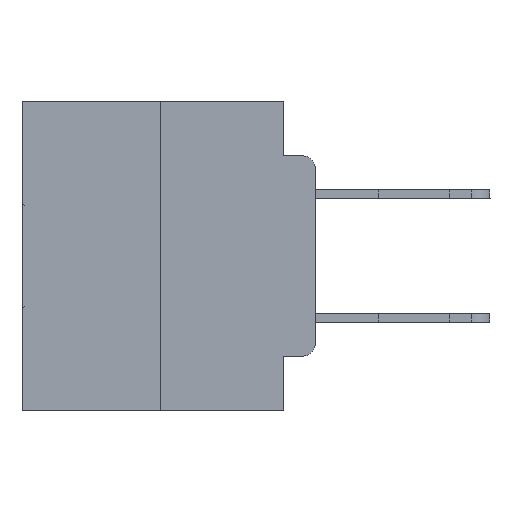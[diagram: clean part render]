
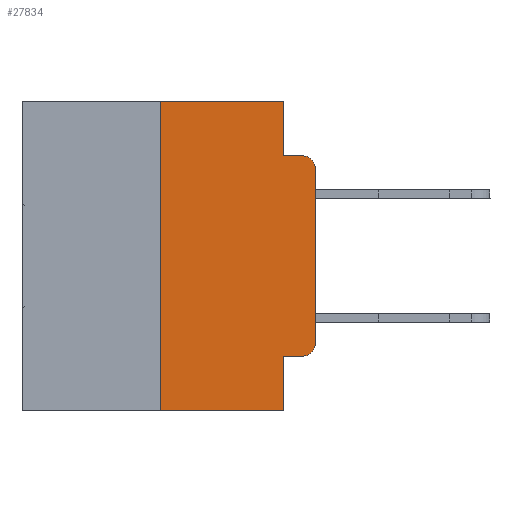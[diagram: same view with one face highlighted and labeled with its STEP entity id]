
A CAD part, left-side view. The second image highlights one B-rep face of the part: STEP entity #27834.
In plain terms, the highlighted planar face has unit normal (-1, 0, 0).
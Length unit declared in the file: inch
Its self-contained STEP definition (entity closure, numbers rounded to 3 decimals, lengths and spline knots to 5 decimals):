
#879 = ORIENTED_EDGE ( 'NONE', *, *, #26324, .F. ) ;
#1026 = FACE_OUTER_BOUND ( 'NONE', #24038, .T. ) ;
#1085 = DIRECTION ( 'NONE',  ( 0., -1., 0. ) ) ;
#1573 = CARTESIAN_POINT ( 'NONE',  ( 0., 0.051, -0.0885 ) ) ;
#1592 = CARTESIAN_POINT ( 'NONE',  ( 0., 0., 0. ) ) ;
#1932 = DIRECTION ( 'NONE',  ( 0., 0., -1. ) ) ;
#1944 = CARTESIAN_POINT ( 'NONE',  ( 0., 0.051, -0.5 ) ) ;
#1952 = CARTESIAN_POINT ( 'NONE',  ( 0., 0.25, -0.5 ) ) ;
#2003 = VERTEX_POINT ( 'NONE', #3719 ) ;
#2290 = VERTEX_POINT ( 'NONE', #1952 ) ;
#2358 = CARTESIAN_POINT ( 'NONE',  ( 0., 0.473, 0. ) ) ;
#2418 = LINE ( 'NONE', #1573, #20305 ) ;
#3221 = CARTESIAN_POINT ( 'NONE',  ( 0., 0.02, -0.4115 ) ) ;
#3252 = AXIS2_PLACEMENT_3D ( 'NONE', #21155, #7186, #23460 ) ;
#3294 = ORIENTED_EDGE ( 'NONE', *, *, #29349, .F. ) ;
#3719 = CARTESIAN_POINT ( 'NONE',  ( 0., 0.25, 0. ) ) ;
#3721 = ORIENTED_EDGE ( 'NONE', *, *, #3937, .F. ) ;
#3920 = DIRECTION ( 'NONE',  ( 0., 0., 1. ) ) ;
#3937 = EDGE_CURVE ( 'NONE', #16353, #20199, #2418, .T. ) ;
#4696 = DIRECTION ( 'NONE',  ( 0., 0., -1. ) ) ;
#5436 = ORIENTED_EDGE ( 'NONE', *, *, #29556, .F. ) ;
#5504 = CARTESIAN_POINT ( 'NONE',  ( 0., 0.02, -0.0885 ) ) ;
#5523 = EDGE_CURVE ( 'NONE', #25826, #20199, #20836, .T. ) ;
#5842 = VECTOR ( 'NONE', #9040, 39.37008 ) ;
#6154 = ORIENTED_EDGE ( 'NONE', *, *, #18633, .T. ) ;
#7186 = DIRECTION ( 'NONE',  ( -1., 0., 0. ) ) ;
#8644 = EDGE_CURVE ( 'NONE', #14102, #25826, #17054, .T. ) ;
#8721 = AXIS2_PLACEMENT_3D ( 'NONE', #29658, #15939, #1932 ) ;
#9040 = DIRECTION ( 'NONE',  ( 0., -1., 0. ) ) ;
#9070 = ORIENTED_EDGE ( 'NONE', *, *, #24800, .F. ) ;
#9284 = DIRECTION ( 'NONE',  ( 0., 0., -1. ) ) ;
#9444 = ORIENTED_EDGE ( 'NONE', *, *, #23275, .T. ) ;
#10222 = CARTESIAN_POINT ( 'NONE',  ( 0., 0.051, -0.4115 ) ) ;
#10243 = ORIENTED_EDGE ( 'NONE', *, *, #5523, .T. ) ;
#10339 = CARTESIAN_POINT ( 'NONE',  ( 0., 0., -0.3915 ) ) ;
#10368 = ORIENTED_EDGE ( 'NONE', *, *, #8644, .T. ) ;
#10516 = VECTOR ( 'NONE', #22574, 39.37008 ) ;
#10648 = EDGE_CURVE ( 'NONE', #2290, #15690, #12847, .T. ) ;
#12090 = CARTESIAN_POINT ( 'NONE',  ( 0., 0.051, 0. ) ) ;
#12847 = LINE ( 'NONE', #20664, #5842 ) ;
#13111 = DIRECTION ( 'NONE',  ( 0., -1., 0. ) ) ;
#13374 = CARTESIAN_POINT ( 'NONE',  ( 0., 0.473, 0. ) ) ;
#14102 = VERTEX_POINT ( 'NONE', #10339 ) ;
#14312 = CARTESIAN_POINT ( 'NONE',  ( 0., 0.051, -0.0885 ) ) ;
#14891 = LINE ( 'NONE', #22088, #26417 ) ;
#15164 = LINE ( 'NONE', #20906, #20594 ) ;
#15690 = VERTEX_POINT ( 'NONE', #1944 ) ;
#15939 = DIRECTION ( 'NONE',  ( -1., 0., 0. ) ) ;
#16353 = VERTEX_POINT ( 'NONE', #14312 ) ;
#17018 = DIRECTION ( 'NONE',  ( 0., 0., -1. ) ) ;
#17054 = LINE ( 'NONE', #1592, #28516 ) ;
#18633 = EDGE_CURVE ( 'NONE', #22022, #14102, #26531, .T. ) ;
#18700 = DIRECTION ( 'NONE',  ( 1., 0., 0. ) ) ;
#19346 = CARTESIAN_POINT ( 'NONE',  ( 0., 0.051, 0. ) ) ;
#19892 = ORIENTED_EDGE ( 'NONE', *, *, #10648, .T. ) ;
#20123 = LINE ( 'NONE', #29163, #25512 ) ;
#20199 = VERTEX_POINT ( 'NONE', #5504 ) ;
#20305 = VECTOR ( 'NONE', #13111, 39.37008 ) ;
#20594 = VECTOR ( 'NONE', #9284, 39.37008 ) ;
#20664 = CARTESIAN_POINT ( 'NONE',  ( 0., 0.473, -0.5 ) ) ;
#20836 = CIRCLE ( 'NONE', #8721, 0.02 ) ;
#20906 = CARTESIAN_POINT ( 'NONE',  ( 0., 0.051, 0. ) ) ;
#20924 = PLANE ( 'NONE',  #26805 ) ;
#21155 = CARTESIAN_POINT ( 'NONE',  ( 0., 0.02, -0.3915 ) ) ;
#21999 = VERTEX_POINT ( 'NONE', #10222 ) ;
#22022 = VERTEX_POINT ( 'NONE', #3221 ) ;
#22088 = CARTESIAN_POINT ( 'NONE',  ( 0., 0.051, -0.4115 ) ) ;
#22574 = DIRECTION ( 'NONE',  ( 0., -1., 0. ) ) ;
#23275 = EDGE_CURVE ( 'NONE', #21999, #22022, #14891, .T. ) ;
#23460 = DIRECTION ( 'NONE',  ( 0., 0., -1. ) ) ;
#24038 = EDGE_LOOP ( 'NONE', ( #10368, #10243, #3721, #3294, #5436, #879, #19892, #9070, #9444, #6154 ) ) ;
#24395 = VERTEX_POINT ( 'NONE', #12090 ) ;
#24800 = EDGE_CURVE ( 'NONE', #21999, #15690, #15164, .T. ) ;
#25512 = VECTOR ( 'NONE', #26906, 39.37008 ) ;
#25826 = VERTEX_POINT ( 'NONE', #27523 ) ;
#26324 = EDGE_CURVE ( 'NONE', #2290, #2003, #20123, .T. ) ;
#26417 = VECTOR ( 'NONE', #1085, 39.37008 ) ;
#26531 = CIRCLE ( 'NONE', #3252, 0.02 ) ;
#26805 = AXIS2_PLACEMENT_3D ( 'NONE', #2358, #18700, #4696 ) ;
#26906 = DIRECTION ( 'NONE',  ( 0., 0., 1. ) ) ;
#27523 = CARTESIAN_POINT ( 'NONE',  ( 0., 0., -0.1085 ) ) ;
#27834 = ADVANCED_FACE ( 'NONE', ( #1026 ), #20924, .F. ) ;
#27850 = VECTOR ( 'NONE', #17018, 39.37008 ) ;
#28183 = LINE ( 'NONE', #13374, #10516 ) ;
#28516 = VECTOR ( 'NONE', #3920, 39.37008 ) ;
#28548 = LINE ( 'NONE', #19346, #27850 ) ;
#29163 = CARTESIAN_POINT ( 'NONE',  ( 0., 0.25, 0. ) ) ;
#29349 = EDGE_CURVE ( 'NONE', #24395, #16353, #28548, .T. ) ;
#29556 = EDGE_CURVE ( 'NONE', #2003, #24395, #28183, .T. ) ;
#29658 = CARTESIAN_POINT ( 'NONE',  ( 0., 0.02, -0.1085 ) ) ;
